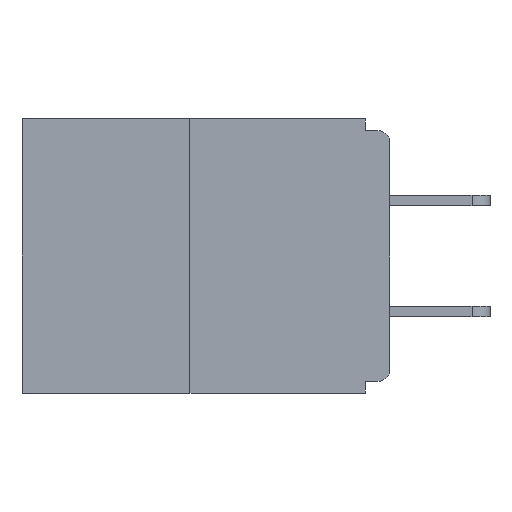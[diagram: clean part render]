
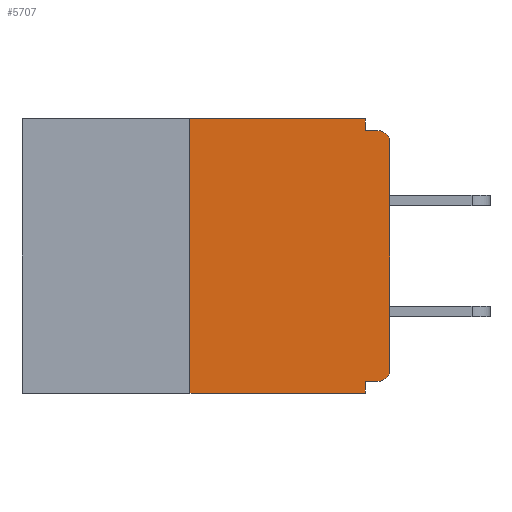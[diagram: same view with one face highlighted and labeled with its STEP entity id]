
A CAD part, left-side view. The second image highlights one B-rep face of the part: STEP entity #5707.
In plain terms, the highlighted planar face has unit normal (-1, 0, 0).
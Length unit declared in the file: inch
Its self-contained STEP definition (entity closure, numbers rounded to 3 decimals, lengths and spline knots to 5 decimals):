
#52 = EDGE_CURVE ( 'NONE', #663, #3145, #4928, .T. ) ;
#151 = LINE ( 'NONE', #13663, #4883 ) ;
#184 = LINE ( 'NONE', #11833, #7101 ) ;
#247 = DIRECTION ( 'NONE',  ( 0., 0., 1. ) ) ;
#365 = LINE ( 'NONE', #9391, #6240 ) ;
#393 = EDGE_CURVE ( 'NONE', #2359, #2684, #184, .T. ) ;
#413 = EDGE_CURVE ( 'NONE', #10655, #10319, #4917, .T. ) ;
#663 = VERTEX_POINT ( 'NONE', #1914 ) ;
#1036 = VECTOR ( 'NONE', #13384, 39.37008 ) ;
#1365 = VECTOR ( 'NONE', #6635, 39.37008 ) ;
#1408 = VECTOR ( 'NONE', #247, 39.37008 ) ;
#1537 = DIRECTION ( 'NONE',  ( -1., 0., 0. ) ) ;
#1765 = AXIS2_PLACEMENT_3D ( 'NONE', #6032, #4100, #5265 ) ;
#1794 = DIRECTION ( 'NONE',  ( 0., -1., 0. ) ) ;
#1914 = CARTESIAN_POINT ( 'NONE',  ( 0., 0.031, -0.328 ) ) ;
#1987 = CARTESIAN_POINT ( 'NONE',  ( 0., 0., -0.313 ) ) ;
#2126 = EDGE_CURVE ( 'NONE', #2359, #3145, #4225, .T. ) ;
#2179 = ORIENTED_EDGE ( 'NONE', *, *, #7688, .F. ) ;
#2350 = AXIS2_PLACEMENT_3D ( 'NONE', #4886, #1537, #11199 ) ;
#2359 = VERTEX_POINT ( 'NONE', #12085 ) ;
#2381 = CARTESIAN_POINT ( 'NONE',  ( 0., 0.031, -0.343 ) ) ;
#2507 = AXIS2_PLACEMENT_3D ( 'NONE', #3442, #10987, #7763 ) ;
#2684 = VERTEX_POINT ( 'NONE', #10393 ) ;
#2691 = CARTESIAN_POINT ( 'NONE',  ( 0., 0.031, -0.015 ) ) ;
#2775 = ORIENTED_EDGE ( 'NONE', *, *, #413, .F. ) ;
#2811 = CIRCLE ( 'NONE', #1765, 0.015 ) ;
#2912 = VECTOR ( 'NONE', #9663, 39.37008 ) ;
#3145 = VERTEX_POINT ( 'NONE', #2381 ) ;
#3294 = DIRECTION ( 'NONE',  ( 0., 0., -1. ) ) ;
#3442 = CARTESIAN_POINT ( 'NONE',  ( 0., 0.46, 0. ) ) ;
#3728 = ORIENTED_EDGE ( 'NONE', *, *, #2126, .T. ) ;
#3935 = ORIENTED_EDGE ( 'NONE', *, *, #13395, .F. ) ;
#4100 = DIRECTION ( 'NONE',  ( -1., 0., 0. ) ) ;
#4150 = CARTESIAN_POINT ( 'NONE',  ( 0., 0., -0.03 ) ) ;
#4195 = VERTEX_POINT ( 'NONE', #1987 ) ;
#4225 = LINE ( 'NONE', #10572, #5403 ) ;
#4395 = CARTESIAN_POINT ( 'NONE',  ( 0., 0., -0.015 ) ) ;
#4883 = VECTOR ( 'NONE', #3294, 39.37008 ) ;
#4886 = CARTESIAN_POINT ( 'NONE',  ( 0., 0.015, -0.03 ) ) ;
#4917 = LINE ( 'NONE', #4395, #1365 ) ;
#4928 = LINE ( 'NONE', #13731, #2912 ) ;
#5265 = DIRECTION ( 'NONE',  ( 0., 0., -1. ) ) ;
#5403 = VECTOR ( 'NONE', #1794, 39.37008 ) ;
#5486 = EDGE_CURVE ( 'NONE', #9389, #4195, #2811, .T. ) ;
#5576 = DIRECTION ( 'NONE',  ( 0., 0., 1. ) ) ;
#5707 = ADVANCED_FACE ( 'NONE', ( #11826 ), #12967, .F. ) ;
#6032 = CARTESIAN_POINT ( 'NONE',  ( 0., 0.015, -0.313 ) ) ;
#6240 = VECTOR ( 'NONE', #13733, 39.37008 ) ;
#6635 = DIRECTION ( 'NONE',  ( 0., -1., 0. ) ) ;
#6684 = EDGE_LOOP ( 'NONE', ( #2179, #8169, #3728, #13442, #3935, #10786, #12315, #11015, #2775, #8800 ) ) ;
#6849 = CIRCLE ( 'NONE', #2350, 0.015 ) ;
#6855 = EDGE_CURVE ( 'NONE', #4195, #12953, #10472, .T. ) ;
#7101 = VECTOR ( 'NONE', #5576, 39.37008 ) ;
#7688 = EDGE_CURVE ( 'NONE', #2684, #11474, #365, .T. ) ;
#7763 = DIRECTION ( 'NONE',  ( 0., 0., -1. ) ) ;
#8169 = ORIENTED_EDGE ( 'NONE', *, *, #393, .F. ) ;
#8437 = EDGE_CURVE ( 'NONE', #11474, #10655, #151, .T. ) ;
#8648 = CARTESIAN_POINT ( 'NONE',  ( 0., 0.031, 0. ) ) ;
#8800 = ORIENTED_EDGE ( 'NONE', *, *, #8437, .F. ) ;
#9029 = CARTESIAN_POINT ( 'NONE',  ( 0., 0.015, -0.328 ) ) ;
#9389 = VERTEX_POINT ( 'NONE', #9029 ) ;
#9391 = CARTESIAN_POINT ( 'NONE',  ( 0., 0.46, 0. ) ) ;
#9663 = DIRECTION ( 'NONE',  ( 0., 0., -1. ) ) ;
#9878 = CARTESIAN_POINT ( 'NONE',  ( 0., 0., 0. ) ) ;
#10319 = VERTEX_POINT ( 'NONE', #10975 ) ;
#10393 = CARTESIAN_POINT ( 'NONE',  ( 0., 0.25, 0. ) ) ;
#10472 = LINE ( 'NONE', #9878, #1408 ) ;
#10572 = CARTESIAN_POINT ( 'NONE',  ( 0., 0.46, -0.343 ) ) ;
#10638 = EDGE_CURVE ( 'NONE', #12953, #10319, #6849, .T. ) ;
#10655 = VERTEX_POINT ( 'NONE', #2691 ) ;
#10786 = ORIENTED_EDGE ( 'NONE', *, *, #5486, .T. ) ;
#10975 = CARTESIAN_POINT ( 'NONE',  ( 0., 0.015, -0.015 ) ) ;
#10987 = DIRECTION ( 'NONE',  ( 1., 0., 0. ) ) ;
#11015 = ORIENTED_EDGE ( 'NONE', *, *, #10638, .T. ) ;
#11199 = DIRECTION ( 'NONE',  ( 0., 0., -1. ) ) ;
#11474 = VERTEX_POINT ( 'NONE', #8648 ) ;
#11826 = FACE_OUTER_BOUND ( 'NONE', #6684, .T. ) ;
#11833 = CARTESIAN_POINT ( 'NONE',  ( 0., 0.25, 0. ) ) ;
#12085 = CARTESIAN_POINT ( 'NONE',  ( 0., 0.25, -0.343 ) ) ;
#12139 = CARTESIAN_POINT ( 'NONE',  ( 0., 0., -0.328 ) ) ;
#12315 = ORIENTED_EDGE ( 'NONE', *, *, #6855, .T. ) ;
#12443 = LINE ( 'NONE', #12139, #1036 ) ;
#12953 = VERTEX_POINT ( 'NONE', #4150 ) ;
#12967 = PLANE ( 'NONE',  #2507 ) ;
#13384 = DIRECTION ( 'NONE',  ( 0., 1., 0. ) ) ;
#13395 = EDGE_CURVE ( 'NONE', #9389, #663, #12443, .T. ) ;
#13442 = ORIENTED_EDGE ( 'NONE', *, *, #52, .F. ) ;
#13663 = CARTESIAN_POINT ( 'NONE',  ( 0., 0.031, 0. ) ) ;
#13731 = CARTESIAN_POINT ( 'NONE',  ( 0., 0.031, -0.343 ) ) ;
#13733 = DIRECTION ( 'NONE',  ( 0., -1., 0. ) ) ;
